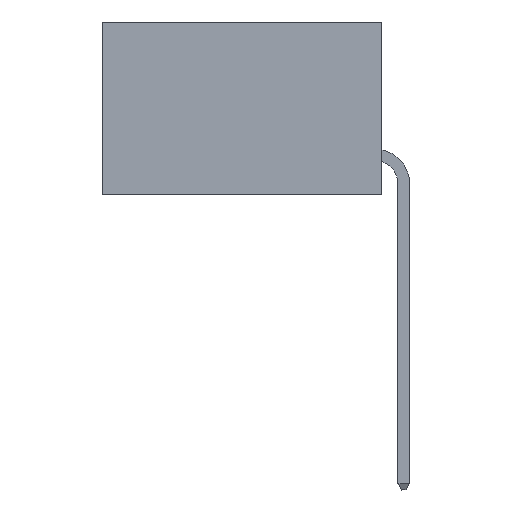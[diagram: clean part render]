
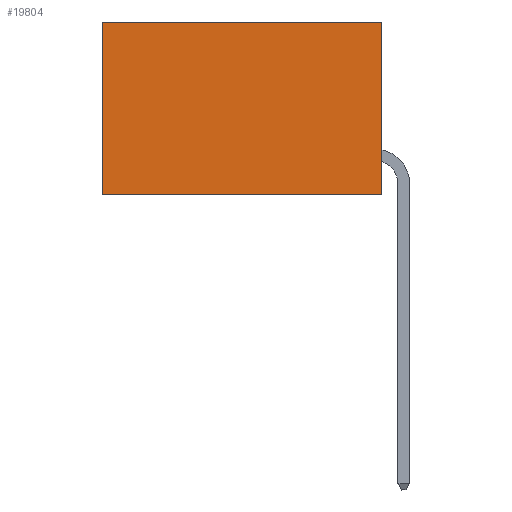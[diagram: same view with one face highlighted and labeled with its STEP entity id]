
A CAD part, left-side view. The second image highlights one B-rep face of the part: STEP entity #19804.
In plain terms, the highlighted planar face has unit normal (-1, 0, 0).
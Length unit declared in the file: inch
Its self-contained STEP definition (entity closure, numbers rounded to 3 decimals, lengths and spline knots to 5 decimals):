
#63 = LINE ( 'NONE', #19329, #36501 ) ;
#242 = ORIENTED_EDGE ( 'NONE', *, *, #25597, .T. ) ;
#334 = LINE ( 'NONE', #7447, #21158 ) ;
#664 = VECTOR ( 'NONE', #4464, 39.37008 ) ;
#1494 = CARTESIAN_POINT ( 'NONE',  ( 0.2875, 0., 0. ) ) ;
#2049 = EDGE_CURVE ( 'NONE', #6410, #2289, #63, .T. ) ;
#2289 = VERTEX_POINT ( 'NONE', #26908 ) ;
#4464 = DIRECTION ( 'NONE',  ( 0., 0., -1. ) ) ;
#5858 = VECTOR ( 'NONE', #32988, 39.37008 ) ;
#6410 = VERTEX_POINT ( 'NONE', #33632 ) ;
#6591 = AXIS2_PLACEMENT_3D ( 'NONE', #22565, #13502, #36711 ) ;
#7447 = CARTESIAN_POINT ( 'NONE',  ( 0.2875, 0., 0. ) ) ;
#7624 = LINE ( 'NONE', #1494, #664 ) ;
#7947 = DIRECTION ( 'NONE',  ( 0., 0., -1. ) ) ;
#8787 = EDGE_CURVE ( 'NONE', #22212, #2289, #14651, .T. ) ;
#10211 = CARTESIAN_POINT ( 'NONE',  ( 0.2875, 0., 0. ) ) ;
#13502 = DIRECTION ( 'NONE',  ( 1., 0., 0. ) ) ;
#14639 = VERTEX_POINT ( 'NONE', #10211 ) ;
#14651 = LINE ( 'NONE', #30252, #5858 ) ;
#16292 = EDGE_LOOP ( 'NONE', ( #19607, #37226, #20089, #242 ) ) ;
#19329 = CARTESIAN_POINT ( 'NONE',  ( 0.2875, 0.6, 0. ) ) ;
#19607 = ORIENTED_EDGE ( 'NONE', *, *, #2049, .T. ) ;
#19804 = ADVANCED_FACE ( 'NONE', ( #21569 ), #22180, .F. ) ;
#20089 = ORIENTED_EDGE ( 'NONE', *, *, #29806, .F. ) ;
#21158 = VECTOR ( 'NONE', #32002, 39.37008 ) ;
#21569 = FACE_OUTER_BOUND ( 'NONE', #16292, .T. ) ;
#22180 = PLANE ( 'NONE',  #6591 ) ;
#22212 = VERTEX_POINT ( 'NONE', #24506 ) ;
#22565 = CARTESIAN_POINT ( 'NONE',  ( 0.2875, 0., 0. ) ) ;
#24506 = CARTESIAN_POINT ( 'NONE',  ( 0.2875, 0., -0.37 ) ) ;
#25597 = EDGE_CURVE ( 'NONE', #14639, #6410, #334, .T. ) ;
#26908 = CARTESIAN_POINT ( 'NONE',  ( 0.2875, 0.6, -0.37 ) ) ;
#29806 = EDGE_CURVE ( 'NONE', #14639, #22212, #7624, .T. ) ;
#30252 = CARTESIAN_POINT ( 'NONE',  ( 0.2875, 0., -0.37 ) ) ;
#32002 = DIRECTION ( 'NONE',  ( 0., 1., 0. ) ) ;
#32988 = DIRECTION ( 'NONE',  ( 0., 1., 0. ) ) ;
#33632 = CARTESIAN_POINT ( 'NONE',  ( 0.2875, 0.6, 0. ) ) ;
#36501 = VECTOR ( 'NONE', #7947, 39.37008 ) ;
#36711 = DIRECTION ( 'NONE',  ( 0., 0., -1. ) ) ;
#37226 = ORIENTED_EDGE ( 'NONE', *, *, #8787, .F. ) ;
